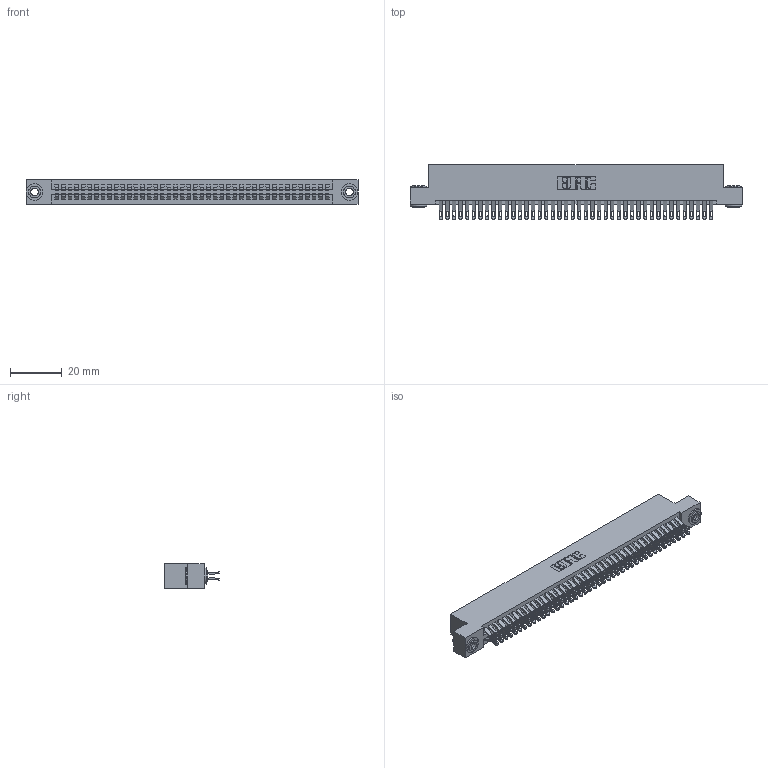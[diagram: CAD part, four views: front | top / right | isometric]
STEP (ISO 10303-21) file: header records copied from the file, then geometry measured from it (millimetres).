
FILE_DESCRIPTION (( 'STEP AP203' ), '1' );
FILE_NAME ('345-084-555-203.STEP', '2018-10-04T02:31:37', ( '' ), ( '' ), 'SwSTEP 2.0', 'SolidWorks 2016', '' );
FILE_SCHEMA (( 'CONFIG_CONTROL_DESIGN' ));
Length unit declared in the file: inch
Products named in the file (4): 345-292-001_555 Tail; 345-084-555-203; 345-250-002_345-250-002-102; 345 Part_Flush Mounting Lugs - 0.156 Dia-TH
Assembly tree (87 placements, depth 2):
  345-084-555-203
    345 Part_Flush Mounting Lugs - 0.156 Dia-TH
    345-292-001_555 Tail  x84
    345-250-002_345-250-002-102  x2
Bounding box: 127.89 x 21.13 x 9.4 mm (x, y, z)
Volume: 12686.3 mm3; surface area: 19804.8 mm2
Topology: 87 solids, 87 shells, 4868 faces, 15285 edges, 10186 vertices
Faces by surface type: plane 2694, cylinder 2166, cone 8
Entity records: 33930 total; most frequent: CARTESIAN_POINT 5697, ORIENTED_EDGE 5594, DIRECTION 5023, EDGE_CURVE 2797, VECTOR 2453, LINE 2453, VERTEX_POINT 1862, AXIS2_PLACEMENT_3D 1285
